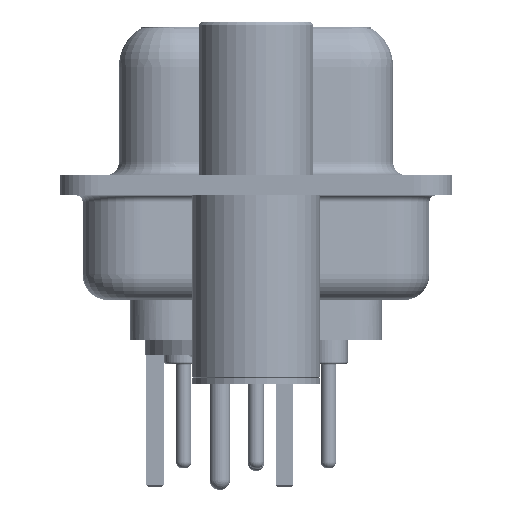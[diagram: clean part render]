
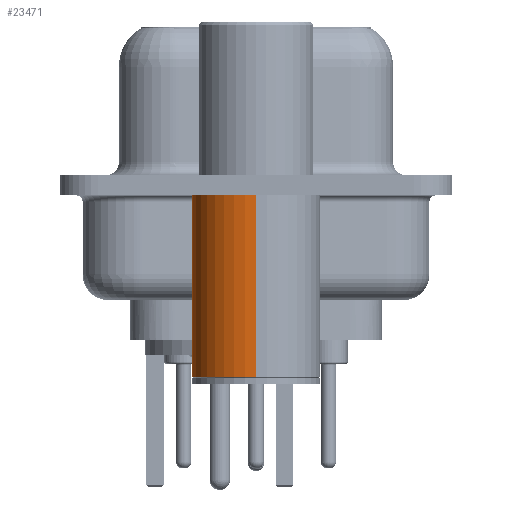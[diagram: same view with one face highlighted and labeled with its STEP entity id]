
A CAD part, left-side view. The second image highlights one B-rep face of the part: STEP entity #23471.
In plain terms, the highlighted cylindrical face has radius 2.5 mm (diameter 5 mm), a partial arc.
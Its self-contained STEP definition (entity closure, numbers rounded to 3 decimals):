
#369 = AXIS2_PLACEMENT_3D ( 'NONE', #24722, #22160, #15889 ) ;
#920 = ORIENTED_EDGE ( 'NONE', *, *, #7107, .T. ) ;
#1147 = DIRECTION ( 'NONE',  ( 1., 0., 0. ) ) ;
#1976 = DIRECTION ( 'NONE',  ( 0., 0., 1. ) ) ;
#3103 = CARTESIAN_POINT ( 'NONE',  ( 0., 0., 0.581 ) ) ;
#3219 = LINE ( 'NONE', #26024, #16110 ) ;
#3425 = CYLINDRICAL_SURFACE ( 'NONE', #32175, 2.5 ) ;
#3461 = ORIENTED_EDGE ( 'NONE', *, *, #16436, .F. ) ;
#5383 = CARTESIAN_POINT ( 'NONE',  ( 2.5, 0., -7.525 ) ) ;
#6913 = EDGE_CURVE ( 'NONE', #11769, #28973, #14994, .T. ) ;
#7107 = EDGE_CURVE ( 'NONE', #33853, #33934, #3219, .T. ) ;
#8343 = ORIENTED_EDGE ( 'NONE', *, *, #6913, .F. ) ;
#11769 = VERTEX_POINT ( 'NONE', #5383 ) ;
#12079 = CARTESIAN_POINT ( 'NONE',  ( -2.5, 0., -7.525 ) ) ;
#12329 = CARTESIAN_POINT ( 'NONE',  ( -2.5, 0., -0.4 ) ) ;
#14446 = DIRECTION ( 'NONE',  ( 0., 0., 1. ) ) ;
#14994 = LINE ( 'NONE', #19349, #35206 ) ;
#15889 = DIRECTION ( 'NONE',  ( 1., 0., 0. ) ) ;
#16110 = VECTOR ( 'NONE', #14446, 1000. ) ;
#16436 = EDGE_CURVE ( 'NONE', #28973, #33934, #33487, .T. ) ;
#17618 = AXIS2_PLACEMENT_3D ( 'NONE', #30350, #18662, #1147 ) ;
#18662 = DIRECTION ( 'NONE',  ( 0., 0., 1. ) ) ;
#19349 = CARTESIAN_POINT ( 'NONE',  ( 2.5, 0., 0.581 ) ) ;
#22160 = DIRECTION ( 'NONE',  ( 0., 0., 1. ) ) ;
#23293 = DIRECTION ( 'NONE',  ( 0., 0., 1. ) ) ;
#23471 = ADVANCED_FACE ( 'NONE', ( #32904 ), #3425, .T. ) ;
#24247 = CARTESIAN_POINT ( 'NONE',  ( 2.5, 0., -0.4 ) ) ;
#24722 = CARTESIAN_POINT ( 'NONE',  ( 0., 0., -7.525 ) ) ;
#24877 = CIRCLE ( 'NONE', #369, 2.5 ) ;
#25270 = ORIENTED_EDGE ( 'NONE', *, *, #32877, .T. ) ;
#26024 = CARTESIAN_POINT ( 'NONE',  ( -2.5, 0., 0.581 ) ) ;
#28149 = EDGE_LOOP ( 'NONE', ( #25270, #920, #3461, #8343 ) ) ;
#28973 = VERTEX_POINT ( 'NONE', #24247 ) ;
#30350 = CARTESIAN_POINT ( 'NONE',  ( 0., 0., -0.4 ) ) ;
#32059 = DIRECTION ( 'NONE',  ( 1., 0., 0. ) ) ;
#32175 = AXIS2_PLACEMENT_3D ( 'NONE', #3103, #23293, #32059 ) ;
#32877 = EDGE_CURVE ( 'NONE', #11769, #33853, #24877, .T. ) ;
#32904 = FACE_OUTER_BOUND ( 'NONE', #28149, .T. ) ;
#33487 = CIRCLE ( 'NONE', #17618, 2.5 ) ;
#33853 = VERTEX_POINT ( 'NONE', #12079 ) ;
#33934 = VERTEX_POINT ( 'NONE', #12329 ) ;
#35206 = VECTOR ( 'NONE', #1976, 1000. ) ;
